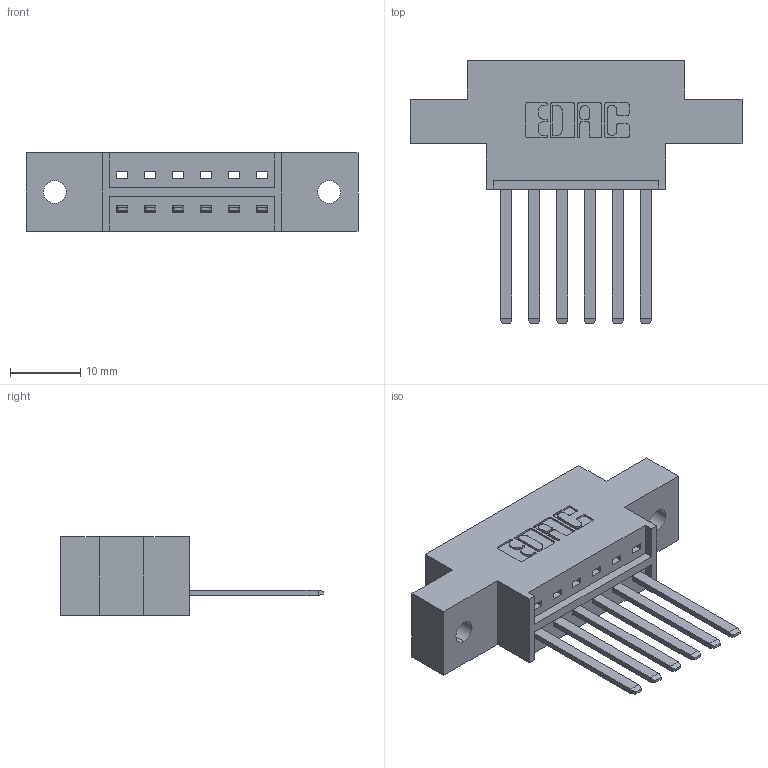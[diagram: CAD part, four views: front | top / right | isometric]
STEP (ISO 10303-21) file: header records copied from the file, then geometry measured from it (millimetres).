
FILE_DESCRIPTION (( 'STEP AP203' ), '1' );
FILE_NAME ('336-006-541-602.STEP', '2020-08-07T19:11:21', ( '' ), ( '' ), 'SwSTEP 2.0', 'SolidWorks 2020', '' );
FILE_SCHEMA (( 'CONFIG_CONTROL_DESIGN' ));
Length unit declared in the file: inch
Products named in the file (3): 336-290-001_336-290-541; 336 Part_Offset - .128 Dia; 336-006-541-602
Assembly tree (7 placements, depth 2):
  336-006-541-602
    336 Part_Offset - .128 Dia
    336-290-001_336-290-541  x6
Bounding box: 47.17 x 37.34 x 11.1 mm (x, y, z)
Volume: 5652.2 mm3; surface area: 5607 mm2
Topology: 7 solids, 7 shells, 418 faces, 1247 edges, 826 vertices
Faces by surface type: plane 278, cylinder 140
Entity records: 8970 total; most frequent: CARTESIAN_POINT 1651, ORIENTED_EDGE 1494, DIRECTION 1367, EDGE_CURVE 747, VECTOR 615, LINE 615, VERTEX_POINT 496, AXIS2_PLACEMENT_3D 376
